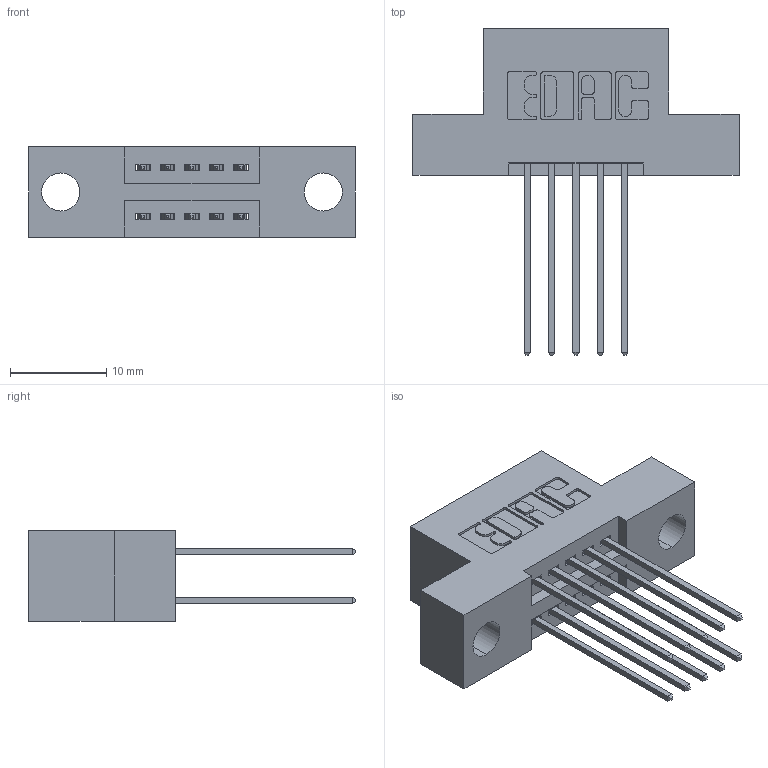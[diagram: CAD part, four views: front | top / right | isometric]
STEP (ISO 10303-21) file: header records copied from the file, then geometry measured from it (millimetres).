
FILE_DESCRIPTION (( 'STEP AP203' ), '1' );
FILE_NAME ('345-010-541-204.STEP', '2021-05-19T15:28:03', ( '' ), ( '' ), 'SwSTEP 2.0', 'SolidWorks 2020', '' );
FILE_SCHEMA (( 'CONFIG_CONTROL_DESIGN' ));
Length unit declared in the file: inch
Products named in the file (3): 345 Part_Flush Mounting Lugs - 0.156 Dia-TI; 345-292-001_345-293-141; 345-010-541-204
Assembly tree (11 placements, depth 2):
  345-010-541-204
    345 Part_Flush Mounting Lugs - 0.156 Dia-TI
    345-292-001_345-293-141  x10
Bounding box: 33.91 x 33.96 x 9.4 mm (x, y, z)
Volume: 2901.9 mm3; surface area: 3694.2 mm2
Topology: 11 solids, 11 shells, 640 faces, 1867 edges, 1230 vertices
Faces by surface type: plane 424, cylinder 216
Entity records: 9341 total; most frequent: CARTESIAN_POINT 1606, ORIENTED_EDGE 1538, DIRECTION 1461, EDGE_CURVE 769, LINE 617, VECTOR 617, VERTEX_POINT 510, AXIS2_PLACEMENT_3D 422
